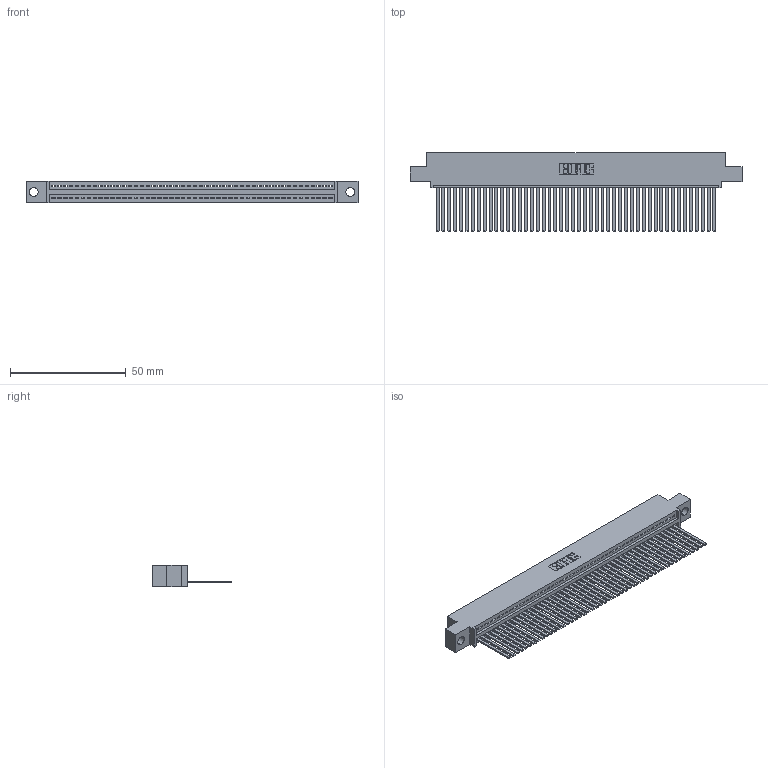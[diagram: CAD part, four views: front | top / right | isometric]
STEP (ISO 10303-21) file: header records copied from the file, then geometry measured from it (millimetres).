
FILE_DESCRIPTION (( 'STEP AP203' ), '1' );
FILE_NAME ('395-048-544-404.STEP', '2021-05-31T15:17:59', ( '' ), ( '' ), 'SwSTEP 2.0', 'SolidWorks 2020', '' );
FILE_SCHEMA (( 'CONFIG_CONTROL_DESIGN' ));
Length unit declared in the file: inch
Products named in the file (3): 345 Part_0.110 Offset - 0.156 Dia-TI; 395-048-544-404; 345-292-001_345-293-144
Assembly tree (49 placements, depth 2):
  395-048-544-404
    345 Part_0.110 Offset - 0.156 Dia-TI
    345-292-001_345-293-144  x48
Bounding box: 143.13 x 33.96 x 9.4 mm (x, y, z)
Volume: 14020.3 mm3; surface area: 20306.5 mm2
Topology: 49 solids, 49 shells, 2640 faces, 7973 edges, 5250 vertices
Faces by surface type: plane 1826, cylinder 814
Entity records: 35685 total; most frequent: CARTESIAN_POINT 6190, ORIENTED_EDGE 6170, DIRECTION 5393, EDGE_CURVE 3085, VECTOR 2765, LINE 2765, VERTEX_POINT 2054, AXIS2_PLACEMENT_3D 1314
